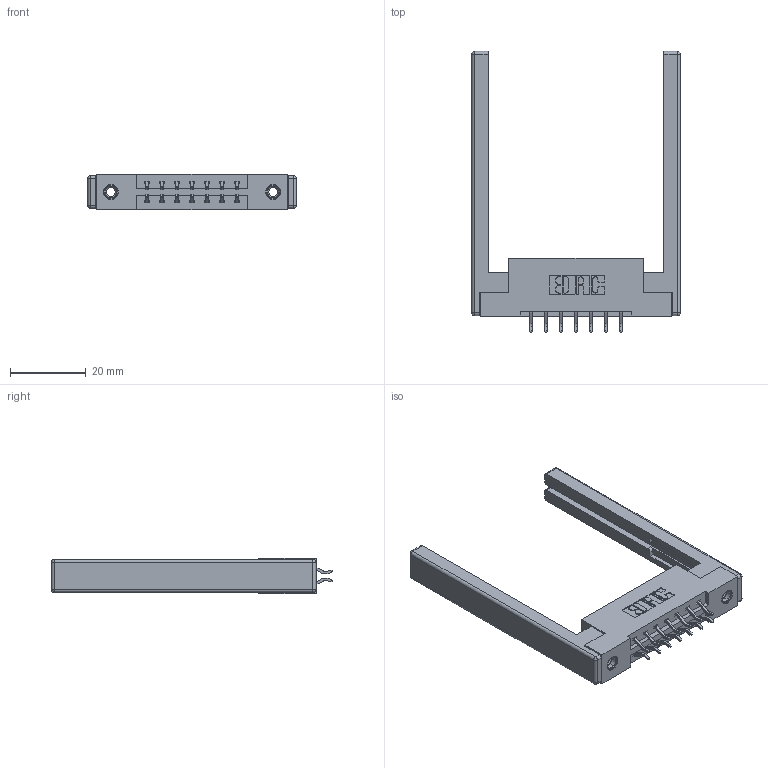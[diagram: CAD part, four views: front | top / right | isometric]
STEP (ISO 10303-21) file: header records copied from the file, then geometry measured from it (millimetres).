
FILE_DESCRIPTION (( 'STEP AP203' ), '1' );
FILE_NAME ('337-014-556-268.STEP', '2019-10-08T11:59:29', ( '' ), ( '' ), 'SwSTEP 2.0', 'SolidWorks 2016', '' );
FILE_SCHEMA (( 'CONFIG_CONTROL_DESIGN' ));
Length unit declared in the file: inch
Products named in the file (5): 337 Part_Flush Mounting Lugs - 0.156 Dia-TI; 345-250-001_345-250-001-102; 337-014-556-268; 307-220-068; 345-292-001_556 Tail
Assembly tree (19 placements, depth 2):
  337-014-556-268
    337 Part_Flush Mounting Lugs - 0.156 Dia-TI
    345-292-001_556 Tail  x14
    345-250-001_345-250-001-102  x2
    307-220-068  x2
Bounding box: 55.17 x 74.31 x 9.4 mm (x, y, z)
Volume: 9732.5 mm3; surface area: 9725.2 mm2
Topology: 19 solids, 19 shells, 1108 faces, 3207 edges, 2098 vertices
Faces by surface type: plane 746, cylinder 338, cone 12, sphere 8, torus 4
Entity records: 12934 total; most frequent: CARTESIAN_POINT 2187, ORIENTED_EDGE 2100, DIRECTION 1984, EDGE_CURVE 1050, LINE 864, VECTOR 864, VERTEX_POINT 690, AXIS2_PLACEMENT_3D 560
